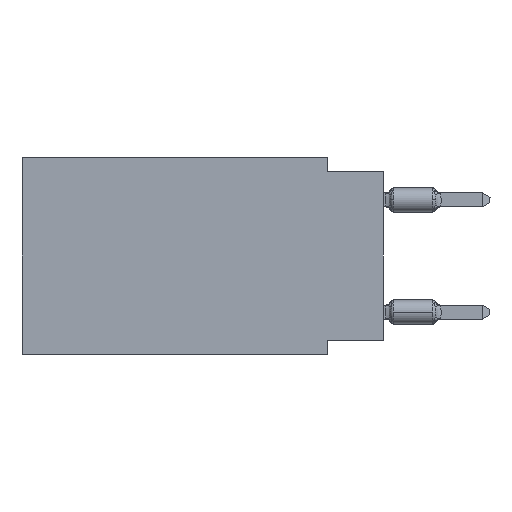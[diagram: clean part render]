
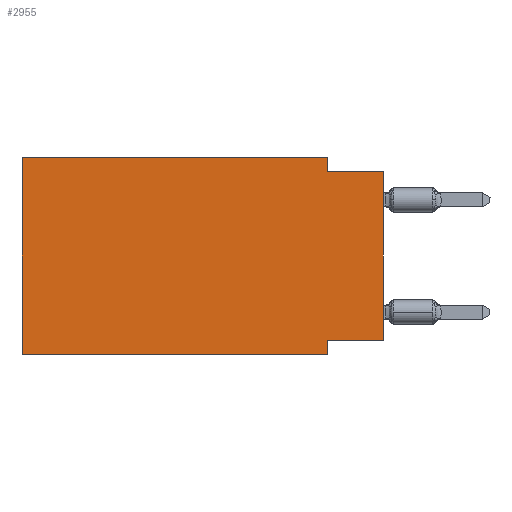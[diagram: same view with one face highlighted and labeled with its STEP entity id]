
A CAD part, left-side view. The second image highlights one B-rep face of the part: STEP entity #2955.
In plain terms, the highlighted planar face has unit normal (-1, 0, 0).
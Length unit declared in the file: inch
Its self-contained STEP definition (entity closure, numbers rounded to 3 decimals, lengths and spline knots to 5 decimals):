
#1040 = DIRECTION ( 'NONE',  ( 0., 0., 1. ) ) ;
#1180 = DIRECTION ( 'NONE',  ( 0., 0., -1. ) ) ;
#1292 = EDGE_CURVE ( 'NONE', #14829, #5540, #19603, .T. ) ;
#1382 = LINE ( 'NONE', #8114, #8007 ) ;
#1771 = CARTESIAN_POINT ( 'NONE',  ( 0., 0.645, 0. ) ) ;
#1880 = EDGE_CURVE ( 'NONE', #14829, #5388, #16910, .T. ) ;
#2955 = ADVANCED_FACE ( 'NONE', ( #11064 ), #6298, .F. ) ;
#3000 = EDGE_CURVE ( 'NONE', #5388, #6343, #9947, .T. ) ;
#4195 = VERTEX_POINT ( 'NONE', #17016 ) ;
#4429 = CARTESIAN_POINT ( 'NONE',  ( 0., 0.645, 0. ) ) ;
#4746 = DIRECTION ( 'NONE',  ( 0., -1., 0. ) ) ;
#5383 = EDGE_CURVE ( 'NONE', #4195, #8418, #19600, .T. ) ;
#5388 = VERTEX_POINT ( 'NONE', #7780 ) ;
#5540 = VERTEX_POINT ( 'NONE', #9983 ) ;
#5571 = VECTOR ( 'NONE', #12649, 39.37008 ) ;
#5902 = CARTESIAN_POINT ( 'NONE',  ( 0., 0., -0.325 ) ) ;
#6041 = CARTESIAN_POINT ( 'NONE',  ( 0., 0.1, -0.025 ) ) ;
#6058 = VECTOR ( 'NONE', #13071, 39.37008 ) ;
#6298 = PLANE ( 'NONE',  #10348 ) ;
#6343 = VERTEX_POINT ( 'NONE', #8266 ) ;
#6555 = CARTESIAN_POINT ( 'NONE',  ( 0., 0.645, -0.35 ) ) ;
#7111 = VERTEX_POINT ( 'NONE', #13383 ) ;
#7780 = CARTESIAN_POINT ( 'NONE',  ( 0., 0.645, 0. ) ) ;
#8007 = VECTOR ( 'NONE', #14955, 39.37008 ) ;
#8104 = DIRECTION ( 'NONE',  ( 0., -1., 0. ) ) ;
#8114 = CARTESIAN_POINT ( 'NONE',  ( 0., 0.1, -0.35 ) ) ;
#8146 = VECTOR ( 'NONE', #1180, 39.37008 ) ;
#8242 = ORIENTED_EDGE ( 'NONE', *, *, #10802, .F. ) ;
#8255 = CARTESIAN_POINT ( 'NONE',  ( 0., 0.1, 0. ) ) ;
#8266 = CARTESIAN_POINT ( 'NONE',  ( 0., 0.1, 0. ) ) ;
#8418 = VERTEX_POINT ( 'NONE', #20086 ) ;
#8906 = EDGE_CURVE ( 'NONE', #6343, #13639, #12898, .T. ) ;
#8930 = VECTOR ( 'NONE', #11941, 39.37008 ) ;
#9767 = CARTESIAN_POINT ( 'NONE',  ( 0., 0., 0. ) ) ;
#9947 = LINE ( 'NONE', #11488, #15994 ) ;
#9949 = ORIENTED_EDGE ( 'NONE', *, *, #5383, .T. ) ;
#9983 = CARTESIAN_POINT ( 'NONE',  ( 0., 0.1, -0.35 ) ) ;
#10119 = ORIENTED_EDGE ( 'NONE', *, *, #8906, .F. ) ;
#10348 = AXIS2_PLACEMENT_3D ( 'NONE', #4429, #12725, #15928 ) ;
#10476 = VECTOR ( 'NONE', #8104, 39.37008 ) ;
#10547 = VECTOR ( 'NONE', #1040, 39.37008 ) ;
#10630 = ORIENTED_EDGE ( 'NONE', *, *, #1880, .F. ) ;
#10802 = EDGE_CURVE ( 'NONE', #4195, #7111, #12754, .T. ) ;
#10913 = ORIENTED_EDGE ( 'NONE', *, *, #21087, .F. ) ;
#11064 = FACE_OUTER_BOUND ( 'NONE', #14169, .T. ) ;
#11373 = ORIENTED_EDGE ( 'NONE', *, *, #3000, .F. ) ;
#11488 = CARTESIAN_POINT ( 'NONE',  ( 0., 0.645, 0. ) ) ;
#11508 = ORIENTED_EDGE ( 'NONE', *, *, #1292, .T. ) ;
#11941 = DIRECTION ( 'NONE',  ( 0., 0., 1. ) ) ;
#12649 = DIRECTION ( 'NONE',  ( 0., 1., 0. ) ) ;
#12725 = DIRECTION ( 'NONE',  ( 1., 0., 0. ) ) ;
#12754 = LINE ( 'NONE', #5902, #5571 ) ;
#12859 = LINE ( 'NONE', #21481, #6058 ) ;
#12898 = LINE ( 'NONE', #8255, #8146 ) ;
#13071 = DIRECTION ( 'NONE',  ( 0., -1., 0. ) ) ;
#13383 = CARTESIAN_POINT ( 'NONE',  ( 0., 0.1, -0.325 ) ) ;
#13639 = VERTEX_POINT ( 'NONE', #6041 ) ;
#14169 = EDGE_LOOP ( 'NONE', ( #9949, #19138, #10119, #11373, #10630, #11508, #10913, #8242 ) ) ;
#14829 = VERTEX_POINT ( 'NONE', #19792 ) ;
#14955 = DIRECTION ( 'NONE',  ( 0., 0., -1. ) ) ;
#15928 = DIRECTION ( 'NONE',  ( 0., 0., -1. ) ) ;
#15994 = VECTOR ( 'NONE', #4746, 39.37008 ) ;
#16910 = LINE ( 'NONE', #1771, #8930 ) ;
#17016 = CARTESIAN_POINT ( 'NONE',  ( 0., 0., -0.325 ) ) ;
#18538 = EDGE_CURVE ( 'NONE', #13639, #8418, #12859, .T. ) ;
#19138 = ORIENTED_EDGE ( 'NONE', *, *, #18538, .F. ) ;
#19600 = LINE ( 'NONE', #9767, #10547 ) ;
#19603 = LINE ( 'NONE', #6555, #10476 ) ;
#19792 = CARTESIAN_POINT ( 'NONE',  ( 0., 0.645, -0.35 ) ) ;
#20086 = CARTESIAN_POINT ( 'NONE',  ( 0., 0., -0.025 ) ) ;
#21087 = EDGE_CURVE ( 'NONE', #7111, #5540, #1382, .T. ) ;
#21481 = CARTESIAN_POINT ( 'NONE',  ( 0., 0., -0.025 ) ) ;
